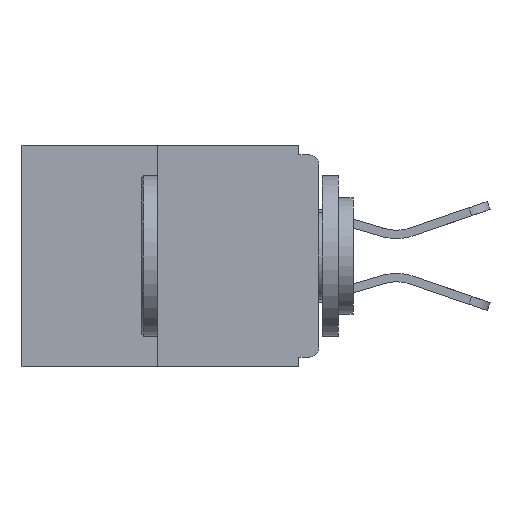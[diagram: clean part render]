
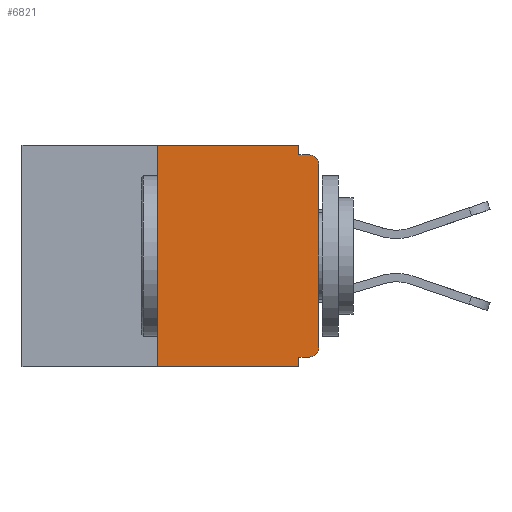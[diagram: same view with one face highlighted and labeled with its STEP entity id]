
A CAD part, left-side view. The second image highlights one B-rep face of the part: STEP entity #6821.
In plain terms, the highlighted planar face has unit normal (-1, 0, 0).
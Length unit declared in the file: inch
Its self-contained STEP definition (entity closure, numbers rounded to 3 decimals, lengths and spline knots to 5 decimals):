
#605 = DIRECTION ( 'NONE',  ( 0., 0., 1. ) ) ;
#729 = DIRECTION ( 'NONE',  ( -1., 0., 0. ) ) ;
#734 = LINE ( 'NONE', #22477, #8846 ) ;
#959 = EDGE_CURVE ( 'NONE', #1158, #1379, #734, .T. ) ;
#1024 = VERTEX_POINT ( 'NONE', #1349 ) ;
#1147 = EDGE_CURVE ( 'NONE', #24900, #13557, #25368, .T. ) ;
#1158 = VERTEX_POINT ( 'NONE', #8425 ) ;
#1349 = CARTESIAN_POINT ( 'NONE',  ( 0., 0.031, -0.343 ) ) ;
#1379 = VERTEX_POINT ( 'NONE', #23881 ) ;
#1581 = ORIENTED_EDGE ( 'NONE', *, *, #8018, .T. ) ;
#1960 = EDGE_CURVE ( 'NONE', #11173, #23645, #22176, .T. ) ;
#1962 = CARTESIAN_POINT ( 'NONE',  ( 0., 0., -0.328 ) ) ;
#2261 = EDGE_CURVE ( 'NONE', #1379, #21177, #16390, .T. ) ;
#2443 = LINE ( 'NONE', #8493, #2790 ) ;
#2790 = VECTOR ( 'NONE', #4216, 39.37008 ) ;
#2958 = CARTESIAN_POINT ( 'NONE',  ( 0., 0.031, 0. ) ) ;
#3006 = DIRECTION ( 'NONE',  ( 0., -1., 0. ) ) ;
#3009 = CARTESIAN_POINT ( 'NONE',  ( 0., 0.015, -0.328 ) ) ;
#4216 = DIRECTION ( 'NONE',  ( 0., 0., 1. ) ) ;
#4249 = EDGE_CURVE ( 'NONE', #12044, #1158, #2443, .T. ) ;
#5676 = CARTESIAN_POINT ( 'NONE',  ( 0., 0.015, -0.015 ) ) ;
#6326 = DIRECTION ( 'NONE',  ( 0., 0., -1. ) ) ;
#6821 = ADVANCED_FACE ( 'NONE', ( #24924 ), #26872, .F. ) ;
#6947 = ORIENTED_EDGE ( 'NONE', *, *, #1147, .T. ) ;
#7519 = LINE ( 'NONE', #25701, #21020 ) ;
#7650 = VECTOR ( 'NONE', #14876, 39.37008 ) ;
#8005 = CARTESIAN_POINT ( 'NONE',  ( 0., 0., -0.313 ) ) ;
#8018 = EDGE_CURVE ( 'NONE', #12044, #1024, #20074, .T. ) ;
#8425 = CARTESIAN_POINT ( 'NONE',  ( 0., 0.25, 0. ) ) ;
#8493 = CARTESIAN_POINT ( 'NONE',  ( 0., 0.25, 0. ) ) ;
#8846 = VECTOR ( 'NONE', #24616, 39.37008 ) ;
#9282 = EDGE_CURVE ( 'NONE', #23645, #1024, #23047, .T. ) ;
#9627 = CARTESIAN_POINT ( 'NONE',  ( 0., 0.46, 0. ) ) ;
#10899 = CARTESIAN_POINT ( 'NONE',  ( 0., 0.015, -0.03 ) ) ;
#11173 = VERTEX_POINT ( 'NONE', #3009 ) ;
#11881 = ORIENTED_EDGE ( 'NONE', *, *, #21336, .T. ) ;
#12044 = VERTEX_POINT ( 'NONE', #23099 ) ;
#12494 = ORIENTED_EDGE ( 'NONE', *, *, #2261, .F. ) ;
#12609 = VECTOR ( 'NONE', #12977, 39.37008 ) ;
#12977 = DIRECTION ( 'NONE',  ( 0., 0., -1. ) ) ;
#13464 = AXIS2_PLACEMENT_3D ( 'NONE', #10899, #14822, #6326 ) ;
#13557 = VERTEX_POINT ( 'NONE', #5676 ) ;
#13653 = CARTESIAN_POINT ( 'NONE',  ( 0., 0.015, -0.313 ) ) ;
#14704 = VECTOR ( 'NONE', #3006, 39.37008 ) ;
#14822 = DIRECTION ( 'NONE',  ( -1., 0., 0. ) ) ;
#14876 = DIRECTION ( 'NONE',  ( 0., 1., 0. ) ) ;
#15345 = AXIS2_PLACEMENT_3D ( 'NONE', #9627, #26777, #24598 ) ;
#15610 = AXIS2_PLACEMENT_3D ( 'NONE', #13653, #729, #17714 ) ;
#16185 = CARTESIAN_POINT ( 'NONE',  ( 0., 0.031, -0.328 ) ) ;
#16369 = EDGE_LOOP ( 'NONE', ( #26403, #20463, #1581, #21572, #17516, #22153, #11881, #6947, #25298, #12494 ) ) ;
#16390 = LINE ( 'NONE', #2958, #20763 ) ;
#16639 = DIRECTION ( 'NONE',  ( 0., 0., -1. ) ) ;
#16716 = VERTEX_POINT ( 'NONE', #8005 ) ;
#16776 = CIRCLE ( 'NONE', #15610, 0.015 ) ;
#17487 = CARTESIAN_POINT ( 'NONE',  ( 0., 0.031, -0.343 ) ) ;
#17516 = ORIENTED_EDGE ( 'NONE', *, *, #1960, .F. ) ;
#17714 = DIRECTION ( 'NONE',  ( 0., 0., -1. ) ) ;
#18019 = CARTESIAN_POINT ( 'NONE',  ( 0., 0.46, -0.343 ) ) ;
#18187 = EDGE_CURVE ( 'NONE', #11173, #16716, #16776, .T. ) ;
#18252 = VECTOR ( 'NONE', #605, 39.37008 ) ;
#18942 = DIRECTION ( 'NONE',  ( 0., -1., 0. ) ) ;
#20074 = LINE ( 'NONE', #18019, #14704 ) ;
#20463 = ORIENTED_EDGE ( 'NONE', *, *, #4249, .F. ) ;
#20763 = VECTOR ( 'NONE', #16639, 39.37008 ) ;
#21020 = VECTOR ( 'NONE', #18942, 39.37008 ) ;
#21177 = VERTEX_POINT ( 'NONE', #26343 ) ;
#21336 = EDGE_CURVE ( 'NONE', #16716, #24900, #26674, .T. ) ;
#21529 = CARTESIAN_POINT ( 'NONE',  ( 0., 0., -0.03 ) ) ;
#21572 = ORIENTED_EDGE ( 'NONE', *, *, #9282, .F. ) ;
#22153 = ORIENTED_EDGE ( 'NONE', *, *, #18187, .T. ) ;
#22176 = LINE ( 'NONE', #1962, #7650 ) ;
#22392 = CARTESIAN_POINT ( 'NONE',  ( 0., 0., 0. ) ) ;
#22477 = CARTESIAN_POINT ( 'NONE',  ( 0., 0.46, 0. ) ) ;
#23047 = LINE ( 'NONE', #17487, #12609 ) ;
#23099 = CARTESIAN_POINT ( 'NONE',  ( 0., 0.25, -0.343 ) ) ;
#23645 = VERTEX_POINT ( 'NONE', #16185 ) ;
#23881 = CARTESIAN_POINT ( 'NONE',  ( 0., 0.031, 0. ) ) ;
#24598 = DIRECTION ( 'NONE',  ( 0., 0., -1. ) ) ;
#24616 = DIRECTION ( 'NONE',  ( 0., -1., 0. ) ) ;
#24900 = VERTEX_POINT ( 'NONE', #21529 ) ;
#24924 = FACE_OUTER_BOUND ( 'NONE', #16369, .T. ) ;
#25298 = ORIENTED_EDGE ( 'NONE', *, *, #26204, .F. ) ;
#25368 = CIRCLE ( 'NONE', #13464, 0.015 ) ;
#25701 = CARTESIAN_POINT ( 'NONE',  ( 0., 0., -0.015 ) ) ;
#26204 = EDGE_CURVE ( 'NONE', #21177, #13557, #7519, .T. ) ;
#26343 = CARTESIAN_POINT ( 'NONE',  ( 0., 0.031, -0.015 ) ) ;
#26403 = ORIENTED_EDGE ( 'NONE', *, *, #959, .F. ) ;
#26674 = LINE ( 'NONE', #22392, #18252 ) ;
#26777 = DIRECTION ( 'NONE',  ( 1., 0., 0. ) ) ;
#26872 = PLANE ( 'NONE',  #15345 ) ;
